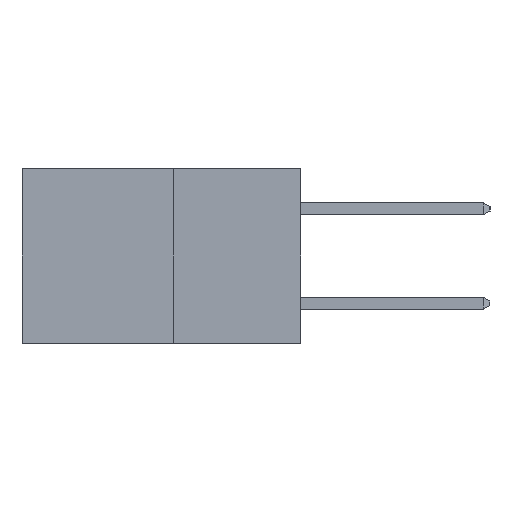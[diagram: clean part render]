
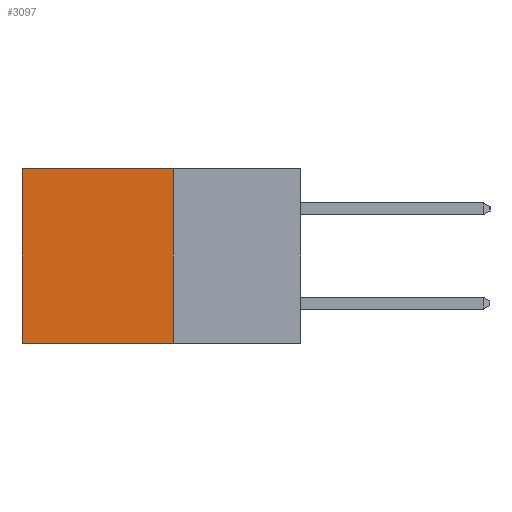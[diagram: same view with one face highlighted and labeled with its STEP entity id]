
A CAD part, left-side view. The second image highlights one B-rep face of the part: STEP entity #3097.
In plain terms, the highlighted planar face has unit normal (-1, 0, 0).
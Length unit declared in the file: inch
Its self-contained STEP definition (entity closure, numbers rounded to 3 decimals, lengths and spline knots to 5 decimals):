
#338 = CARTESIAN_POINT ( 'NONE',  ( 0.277, 0.27, -0.37 ) ) ;
#493 = LINE ( 'NONE', #338, #2765 ) ;
#764 = ORIENTED_EDGE ( 'NONE', *, *, #6594, .F. ) ;
#1226 = ORIENTED_EDGE ( 'NONE', *, *, #9141, .F. ) ;
#1603 = VERTEX_POINT ( 'NONE', #9299 ) ;
#2023 = FACE_OUTER_BOUND ( 'NONE', #8076, .T. ) ;
#2489 = LINE ( 'NONE', #8070, #6245 ) ;
#2765 = VECTOR ( 'NONE', #5670, 39.37008 ) ;
#2827 = VERTEX_POINT ( 'NONE', #3951 ) ;
#3097 = ADVANCED_FACE ( 'NONE', ( #2023 ), #8992, .F. ) ;
#3327 = VECTOR ( 'NONE', #6261, 39.37008 ) ;
#3580 = LINE ( 'NONE', #6328, #3327 ) ;
#3583 = EDGE_CURVE ( 'NONE', #1603, #2827, #3580, .T. ) ;
#3951 = CARTESIAN_POINT ( 'NONE',  ( 0.277, 0.59, 0. ) ) ;
#4545 = DIRECTION ( 'NONE',  ( 0., 0., -1. ) ) ;
#4581 = AXIS2_PLACEMENT_3D ( 'NONE', #8957, #9390, #9031 ) ;
#4748 = VERTEX_POINT ( 'NONE', #6235 ) ;
#4979 = DIRECTION ( 'NONE',  ( 0., 0., -1. ) ) ;
#5670 = DIRECTION ( 'NONE',  ( 0., 1., 0. ) ) ;
#6093 = EDGE_CURVE ( 'NONE', #2827, #4748, #6954, .T. ) ;
#6235 = CARTESIAN_POINT ( 'NONE',  ( 0.277, 0.59, -0.37 ) ) ;
#6245 = VECTOR ( 'NONE', #4545, 39.37008 ) ;
#6261 = DIRECTION ( 'NONE',  ( 0., 1., 0. ) ) ;
#6328 = CARTESIAN_POINT ( 'NONE',  ( 0.277, 0.27, 0. ) ) ;
#6405 = CARTESIAN_POINT ( 'NONE',  ( 0.277, 0.59, -0.37 ) ) ;
#6594 = EDGE_CURVE ( 'NONE', #8987, #4748, #493, .T. ) ;
#6954 = LINE ( 'NONE', #6405, #8768 ) ;
#6976 = ORIENTED_EDGE ( 'NONE', *, *, #3583, .T. ) ;
#8070 = CARTESIAN_POINT ( 'NONE',  ( 0.277, 0.27, -0.37 ) ) ;
#8076 = EDGE_LOOP ( 'NONE', ( #9117, #764, #1226, #6976 ) ) ;
#8615 = CARTESIAN_POINT ( 'NONE',  ( 0.277, 0.27, -0.37 ) ) ;
#8768 = VECTOR ( 'NONE', #4979, 39.37008 ) ;
#8957 = CARTESIAN_POINT ( 'NONE',  ( 0.277, 0.27, -0.37 ) ) ;
#8987 = VERTEX_POINT ( 'NONE', #8615 ) ;
#8992 = PLANE ( 'NONE',  #4581 ) ;
#9031 = DIRECTION ( 'NONE',  ( 0., 0., -1. ) ) ;
#9117 = ORIENTED_EDGE ( 'NONE', *, *, #6093, .T. ) ;
#9141 = EDGE_CURVE ( 'NONE', #1603, #8987, #2489, .T. ) ;
#9299 = CARTESIAN_POINT ( 'NONE',  ( 0.277, 0.27, 0. ) ) ;
#9390 = DIRECTION ( 'NONE',  ( 1., 0., 0. ) ) ;
